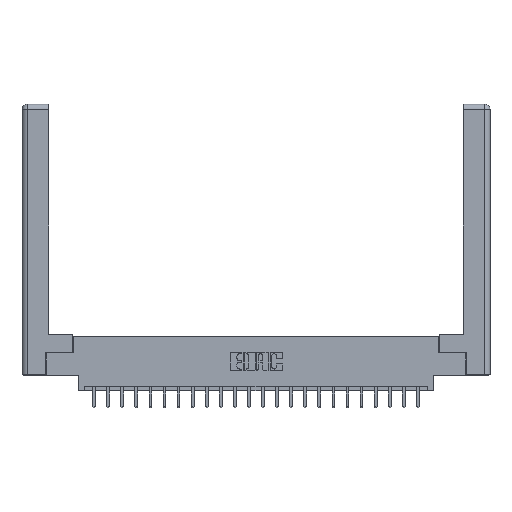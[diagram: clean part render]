
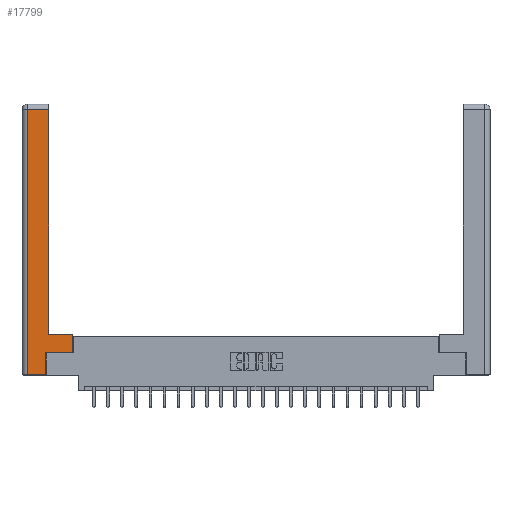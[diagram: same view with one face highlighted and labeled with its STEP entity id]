
A CAD part, top view. The second image highlights one B-rep face of the part: STEP entity #17799.
In plain terms, the highlighted planar face has unit normal (0, 0, 1).
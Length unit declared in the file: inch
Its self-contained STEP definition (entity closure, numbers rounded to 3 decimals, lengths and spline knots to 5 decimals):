
#362 = CARTESIAN_POINT ( 'NONE',  ( 0.565, 0.245, 0. ) ) ;
#1087 = AXIS2_PLACEMENT_3D ( 'NONE', #21822, #14358, #16203 ) ;
#1321 = DIRECTION ( 'NONE',  ( 0., 1., 0. ) ) ;
#2108 = CARTESIAN_POINT ( 'NONE',  ( 0.565, 0.245, 0. ) ) ;
#2362 = DIRECTION ( 'NONE',  ( 0., 1., 0. ) ) ;
#2671 = VECTOR ( 'NONE', #1321, 39.37008 ) ;
#3095 = ORIENTED_EDGE ( 'NONE', *, *, #11135, .T. ) ;
#3159 = CARTESIAN_POINT ( 'NONE',  ( 0.265, 0.245, 0. ) ) ;
#3265 = VECTOR ( 'NONE', #7357, 39.37008 ) ;
#3435 = EDGE_CURVE ( 'NONE', #14106, #9382, #19392, .T. ) ;
#3536 = CARTESIAN_POINT ( 'NONE',  ( 0.0615, 0., 0. ) ) ;
#3542 = LINE ( 'NONE', #23650, #5554 ) ;
#3678 = EDGE_CURVE ( 'NONE', #9382, #17802, #21089, .T. ) ;
#3798 = VECTOR ( 'NONE', #6903, 39.37008 ) ;
#4133 = EDGE_CURVE ( 'NONE', #11407, #14314, #17328, .T. ) ;
#4503 = VERTEX_POINT ( 'NONE', #20401 ) ;
#5076 = ORIENTED_EDGE ( 'NONE', *, *, #4133, .T. ) ;
#5456 = CARTESIAN_POINT ( 'NONE',  ( 0.0615, 2.94, 0. ) ) ;
#5554 = VECTOR ( 'NONE', #12707, 39.37008 ) ;
#5724 = DIRECTION ( 'NONE',  ( 0., 1., 0. ) ) ;
#6326 = LINE ( 'NONE', #17165, #8032 ) ;
#6903 = DIRECTION ( 'NONE',  ( -1., 0., 0. ) ) ;
#6941 = CARTESIAN_POINT ( 'NONE',  ( 0.565, 0.45, 0. ) ) ;
#7284 = CARTESIAN_POINT ( 'NONE',  ( 0.295, 2.94, 0. ) ) ;
#7357 = DIRECTION ( 'NONE',  ( 1., 0., 0. ) ) ;
#7399 = FACE_OUTER_BOUND ( 'NONE', #10704, .T. ) ;
#7716 = LINE ( 'NONE', #10360, #13478 ) ;
#7955 = CARTESIAN_POINT ( 'NONE',  ( 0.0615, 2.94, 0. ) ) ;
#8032 = VECTOR ( 'NONE', #2362, 39.37008 ) ;
#8767 = CARTESIAN_POINT ( 'NONE',  ( 0.565, 0.45, 0. ) ) ;
#8862 = EDGE_CURVE ( 'NONE', #15877, #14106, #13303, .T. ) ;
#9382 = VERTEX_POINT ( 'NONE', #2108 ) ;
#10124 = ORIENTED_EDGE ( 'NONE', *, *, #23498, .T. ) ;
#10198 = DIRECTION ( 'NONE',  ( 1., 0., 0. ) ) ;
#10360 = CARTESIAN_POINT ( 'NONE',  ( 0.265, 0., 0. ) ) ;
#10688 = EDGE_CURVE ( 'NONE', #16937, #11407, #6326, .T. ) ;
#10704 = EDGE_LOOP ( 'NONE', ( #20986, #5076, #22882, #3095, #16169, #18527, #12474, #10124 ) ) ;
#11135 = EDGE_CURVE ( 'NONE', #4503, #15877, #7716, .T. ) ;
#11407 = VERTEX_POINT ( 'NONE', #7284 ) ;
#12474 = ORIENTED_EDGE ( 'NONE', *, *, #3678, .T. ) ;
#12483 = PLANE ( 'NONE',  #1087 ) ;
#12707 = DIRECTION ( 'NONE',  ( -1., 0., 0. ) ) ;
#13303 = LINE ( 'NONE', #18752, #23053 ) ;
#13478 = VECTOR ( 'NONE', #10198, 39.37008 ) ;
#14099 = VECTOR ( 'NONE', #20111, 39.37008 ) ;
#14106 = VERTEX_POINT ( 'NONE', #3159 ) ;
#14314 = VERTEX_POINT ( 'NONE', #7955 ) ;
#14358 = DIRECTION ( 'NONE',  ( 0., 0., -1. ) ) ;
#15877 = VERTEX_POINT ( 'NONE', #19121 ) ;
#16169 = ORIENTED_EDGE ( 'NONE', *, *, #8862, .T. ) ;
#16203 = DIRECTION ( 'NONE',  ( -1., 0., 0. ) ) ;
#16821 = EDGE_CURVE ( 'NONE', #14314, #4503, #20127, .T. ) ;
#16937 = VERTEX_POINT ( 'NONE', #20822 ) ;
#17165 = CARTESIAN_POINT ( 'NONE',  ( 0.295, 3., 0. ) ) ;
#17328 = LINE ( 'NONE', #5456, #3798 ) ;
#17799 = ADVANCED_FACE ( 'NONE', ( #7399 ), #12483, .F. ) ;
#17802 = VERTEX_POINT ( 'NONE', #6941 ) ;
#18527 = ORIENTED_EDGE ( 'NONE', *, *, #3435, .T. ) ;
#18752 = CARTESIAN_POINT ( 'NONE',  ( 0.265, 0.245, 0. ) ) ;
#19121 = CARTESIAN_POINT ( 'NONE',  ( 0.265, 0., 0. ) ) ;
#19392 = LINE ( 'NONE', #362, #3265 ) ;
#20111 = DIRECTION ( 'NONE',  ( 0., -1., 0. ) ) ;
#20127 = LINE ( 'NONE', #3536, #14099 ) ;
#20401 = CARTESIAN_POINT ( 'NONE',  ( 0.0615, 0., 0. ) ) ;
#20822 = CARTESIAN_POINT ( 'NONE',  ( 0.295, 0.45, 0. ) ) ;
#20986 = ORIENTED_EDGE ( 'NONE', *, *, #10688, .T. ) ;
#21089 = LINE ( 'NONE', #8767, #2671 ) ;
#21822 = CARTESIAN_POINT ( 'NONE',  ( 0., 0., 0. ) ) ;
#22882 = ORIENTED_EDGE ( 'NONE', *, *, #16821, .T. ) ;
#23053 = VECTOR ( 'NONE', #5724, 39.37008 ) ;
#23498 = EDGE_CURVE ( 'NONE', #17802, #16937, #3542, .T. ) ;
#23650 = CARTESIAN_POINT ( 'NONE',  ( 0.295, 0.45, 0. ) ) ;
